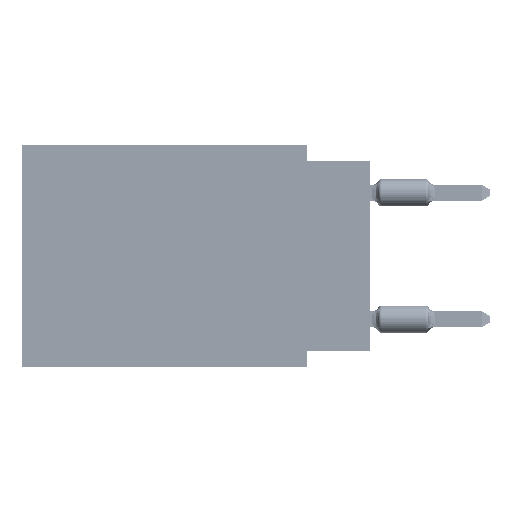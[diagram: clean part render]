
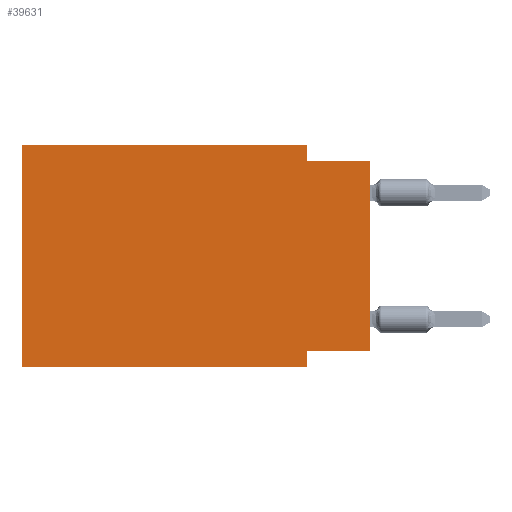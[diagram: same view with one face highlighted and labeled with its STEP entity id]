
A CAD part, left-side view. The second image highlights one B-rep face of the part: STEP entity #39631.
In plain terms, the highlighted planar face has unit normal (-1, 0, 0).
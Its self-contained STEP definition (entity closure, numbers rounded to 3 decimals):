
#507 = VECTOR ( 'NONE', #31075, 1000. ) ;
#4026 = CARTESIAN_POINT ( 'NONE',  ( 0., 0., -8.255 ) ) ;
#4645 = VERTEX_POINT ( 'NONE', #44703 ) ;
#4943 = EDGE_CURVE ( 'NONE', #70396, #18793, #66764, .T. ) ;
#5239 = CARTESIAN_POINT ( 'NONE',  ( 0., 0., -0.635 ) ) ;
#5826 = LINE ( 'NONE', #62760, #30670 ) ;
#6043 = CARTESIAN_POINT ( 'NONE',  ( 0., 13.97, -8.89 ) ) ;
#16665 = ORIENTED_EDGE ( 'NONE', *, *, #22803, .F. ) ;
#17066 = DIRECTION ( 'NONE',  ( 0., 0., -1. ) ) ;
#17933 = VERTEX_POINT ( 'NONE', #60313 ) ;
#18793 = VERTEX_POINT ( 'NONE', #5239 ) ;
#19092 = VERTEX_POINT ( 'NONE', #22678 ) ;
#20197 = LINE ( 'NONE', #47539, #507 ) ;
#20536 = DIRECTION ( 'NONE',  ( 0., -1., 0. ) ) ;
#20837 = EDGE_CURVE ( 'NONE', #17933, #72283, #5826, .T. ) ;
#22678 = CARTESIAN_POINT ( 'NONE',  ( 0., 2.54, 0. ) ) ;
#22803 = EDGE_CURVE ( 'NONE', #25667, #4645, #66902, .T. ) ;
#23271 = LINE ( 'NONE', #6043, #68827 ) ;
#23722 = CARTESIAN_POINT ( 'NONE',  ( 0., 13.97, -8.89 ) ) ;
#24201 = DIRECTION ( 'NONE',  ( 1., 0., 0. ) ) ;
#25667 = VERTEX_POINT ( 'NONE', #23722 ) ;
#26523 = DIRECTION ( 'NONE',  ( 0., 1., 0. ) ) ;
#28048 = AXIS2_PLACEMENT_3D ( 'NONE', #58296, #24201, #29833 ) ;
#29381 = ORIENTED_EDGE ( 'NONE', *, *, #32380, .F. ) ;
#29833 = DIRECTION ( 'NONE',  ( 0., 0., -1. ) ) ;
#30670 = VECTOR ( 'NONE', #17066, 1000. ) ;
#30922 = ORIENTED_EDGE ( 'NONE', *, *, #31412, .F. ) ;
#31075 = DIRECTION ( 'NONE',  ( 0., -1., 0. ) ) ;
#31412 = EDGE_CURVE ( 'NONE', #19092, #59316, #54017, .T. ) ;
#32380 = EDGE_CURVE ( 'NONE', #70396, #17933, #48637, .T. ) ;
#33497 = CARTESIAN_POINT ( 'NONE',  ( 0., 2.54, -8.89 ) ) ;
#34400 = EDGE_CURVE ( 'NONE', #4645, #19092, #48993, .T. ) ;
#35456 = PLANE ( 'NONE',  #28048 ) ;
#38681 = EDGE_CURVE ( 'NONE', #25667, #72283, #23271, .T. ) ;
#38781 = DIRECTION ( 'NONE',  ( 0., 0., 1. ) ) ;
#38785 = EDGE_LOOP ( 'NONE', ( #49345, #55793, #30922, #46163, #16665, #61188, #55986, #29381 ) ) ;
#39631 = ADVANCED_FACE ( 'NONE', ( #46678 ), #35456, .F. ) ;
#40767 = CARTESIAN_POINT ( 'NONE',  ( 0., 0., -8.255 ) ) ;
#42044 = CARTESIAN_POINT ( 'NONE',  ( 0., 2.54, 0. ) ) ;
#42777 = DIRECTION ( 'NONE',  ( 0., 0., -1. ) ) ;
#43523 = DIRECTION ( 'NONE',  ( 0., 0., 1. ) ) ;
#44392 = CARTESIAN_POINT ( 'NONE',  ( 0., 13.97, 0. ) ) ;
#44703 = CARTESIAN_POINT ( 'NONE',  ( 0., 13.97, 0. ) ) ;
#46163 = ORIENTED_EDGE ( 'NONE', *, *, #34400, .F. ) ;
#46678 = FACE_OUTER_BOUND ( 'NONE', #38785, .T. ) ;
#47539 = CARTESIAN_POINT ( 'NONE',  ( 0., 0., -0.635 ) ) ;
#48637 = LINE ( 'NONE', #4026, #50157 ) ;
#48889 = VECTOR ( 'NONE', #42777, 1000. ) ;
#48993 = LINE ( 'NONE', #71876, #54570 ) ;
#49345 = ORIENTED_EDGE ( 'NONE', *, *, #4943, .T. ) ;
#50157 = VECTOR ( 'NONE', #26523, 1000. ) ;
#54017 = LINE ( 'NONE', #42044, #48889 ) ;
#54570 = VECTOR ( 'NONE', #20536, 1000. ) ;
#55793 = ORIENTED_EDGE ( 'NONE', *, *, #59848, .F. ) ;
#55986 = ORIENTED_EDGE ( 'NONE', *, *, #20837, .F. ) ;
#57728 = DIRECTION ( 'NONE',  ( 0., -1., 0. ) ) ;
#58296 = CARTESIAN_POINT ( 'NONE',  ( 0., 13.97, 0. ) ) ;
#59316 = VERTEX_POINT ( 'NONE', #63746 ) ;
#59848 = EDGE_CURVE ( 'NONE', #59316, #18793, #20197, .T. ) ;
#60313 = CARTESIAN_POINT ( 'NONE',  ( 0., 2.54, -8.255 ) ) ;
#61188 = ORIENTED_EDGE ( 'NONE', *, *, #38681, .T. ) ;
#62760 = CARTESIAN_POINT ( 'NONE',  ( 0., 2.54, -8.89 ) ) ;
#63746 = CARTESIAN_POINT ( 'NONE',  ( 0., 2.54, -0.635 ) ) ;
#66764 = LINE ( 'NONE', #71664, #73379 ) ;
#66902 = LINE ( 'NONE', #44392, #70493 ) ;
#68827 = VECTOR ( 'NONE', #57728, 1000. ) ;
#70396 = VERTEX_POINT ( 'NONE', #40767 ) ;
#70493 = VECTOR ( 'NONE', #38781, 1000. ) ;
#71664 = CARTESIAN_POINT ( 'NONE',  ( 0., 0., 0. ) ) ;
#71876 = CARTESIAN_POINT ( 'NONE',  ( 0., 13.97, 0. ) ) ;
#72283 = VERTEX_POINT ( 'NONE', #33497 ) ;
#73379 = VECTOR ( 'NONE', #43523, 1000. ) ;
